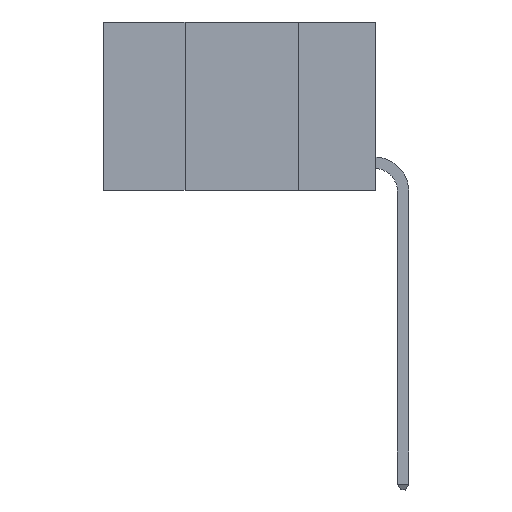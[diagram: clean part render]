
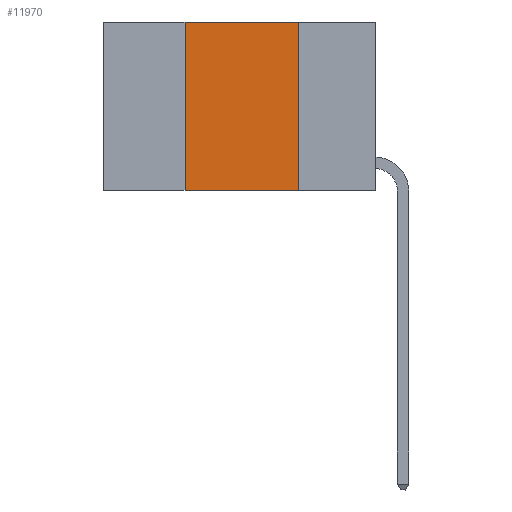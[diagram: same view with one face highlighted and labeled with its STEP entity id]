
A CAD part, left-side view. The second image highlights one B-rep face of the part: STEP entity #11970.
In plain terms, the highlighted planar face has unit normal (-1, 0, 0).
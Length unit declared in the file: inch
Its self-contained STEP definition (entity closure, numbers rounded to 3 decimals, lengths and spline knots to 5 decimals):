
#653 = CARTESIAN_POINT ( 'NONE',  ( 0., 0.6, 0. ) ) ;
#980 = DIRECTION ( 'NONE',  ( 0., -1., 0. ) ) ;
#1029 = FACE_OUTER_BOUND ( 'NONE', #6077, .T. ) ;
#1090 = VECTOR ( 'NONE', #980, 39.37008 ) ;
#1405 = VERTEX_POINT ( 'NONE', #14710 ) ;
#1873 = DIRECTION ( 'NONE',  ( 0., 0., -1. ) ) ;
#2526 = EDGE_CURVE ( 'NONE', #6929, #7351, #3485, .T. ) ;
#3146 = CARTESIAN_POINT ( 'NONE',  ( 0., 0.42, 0. ) ) ;
#3485 = LINE ( 'NONE', #6517, #12460 ) ;
#4108 = EDGE_CURVE ( 'NONE', #8711, #1405, #13979, .T. ) ;
#6077 = EDGE_LOOP ( 'NONE', ( #10921, #11081, #11095, #11210 ) ) ;
#6200 = EDGE_CURVE ( 'NONE', #1405, #6929, #11989, .T. ) ;
#6517 = CARTESIAN_POINT ( 'NONE',  ( 0., 0.17, 0. ) ) ;
#6559 = DIRECTION ( 'NONE',  ( 0., 0., -1. ) ) ;
#6911 = CARTESIAN_POINT ( 'NONE',  ( 0., 0.17, 0. ) ) ;
#6929 = VERTEX_POINT ( 'NONE', #6911 ) ;
#7017 = DIRECTION ( 'NONE',  ( 0., -1., 0. ) ) ;
#7056 = LINE ( 'NONE', #9341, #1090 ) ;
#7351 = VERTEX_POINT ( 'NONE', #12221 ) ;
#8711 = VERTEX_POINT ( 'NONE', #10261 ) ;
#8972 = DIRECTION ( 'NONE',  ( 1., 0., 0. ) ) ;
#9341 = CARTESIAN_POINT ( 'NONE',  ( 0., 0.6, -0.37 ) ) ;
#10034 = VECTOR ( 'NONE', #7017, 39.37008 ) ;
#10141 = EDGE_CURVE ( 'NONE', #8711, #7351, #7056, .T. ) ;
#10220 = DIRECTION ( 'NONE',  ( 0., 0., 1. ) ) ;
#10261 = CARTESIAN_POINT ( 'NONE',  ( 0., 0.42, -0.37 ) ) ;
#10921 = ORIENTED_EDGE ( 'NONE', *, *, #2526, .F. ) ;
#11000 = VECTOR ( 'NONE', #10220, 39.37008 ) ;
#11081 = ORIENTED_EDGE ( 'NONE', *, *, #6200, .F. ) ;
#11095 = ORIENTED_EDGE ( 'NONE', *, *, #4108, .F. ) ;
#11210 = ORIENTED_EDGE ( 'NONE', *, *, #10141, .T. ) ;
#11970 = ADVANCED_FACE ( 'NONE', ( #1029 ), #13524, .F. ) ;
#11989 = LINE ( 'NONE', #13892, #10034 ) ;
#12221 = CARTESIAN_POINT ( 'NONE',  ( 0., 0.17, -0.37 ) ) ;
#12460 = VECTOR ( 'NONE', #6559, 39.37008 ) ;
#12462 = AXIS2_PLACEMENT_3D ( 'NONE', #653, #8972, #1873 ) ;
#13524 = PLANE ( 'NONE',  #12462 ) ;
#13892 = CARTESIAN_POINT ( 'NONE',  ( 0., 0.6, 0. ) ) ;
#13979 = LINE ( 'NONE', #3146, #11000 ) ;
#14710 = CARTESIAN_POINT ( 'NONE',  ( 0., 0.42, 0. ) ) ;
